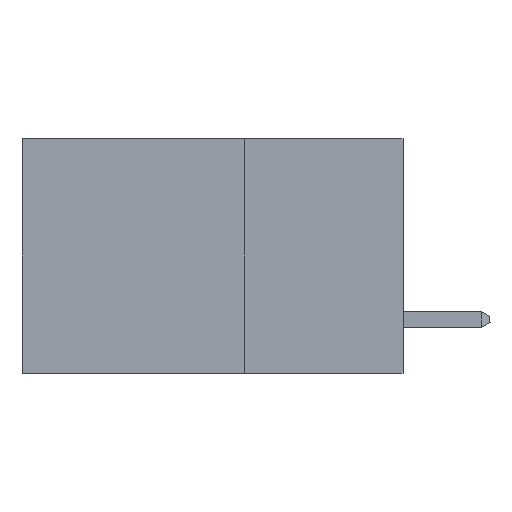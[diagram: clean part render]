
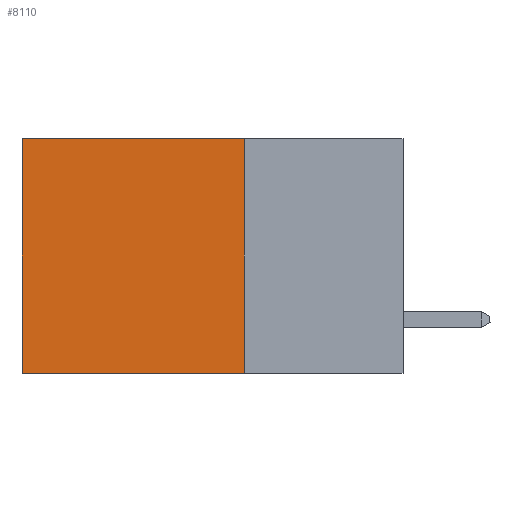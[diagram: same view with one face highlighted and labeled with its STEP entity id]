
A CAD part, left-side view. The second image highlights one B-rep face of the part: STEP entity #8110.
In plain terms, the highlighted planar face has unit normal (-1, 0, 0).
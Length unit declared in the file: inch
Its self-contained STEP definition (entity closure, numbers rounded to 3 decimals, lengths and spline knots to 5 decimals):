
#1140 = EDGE_CURVE ( 'NONE', #17982, #34560, #24422, .T. ) ;
#2813 = CARTESIAN_POINT ( 'NONE',  ( 0.2875, 0.6, -0.37 ) ) ;
#3081 = CARTESIAN_POINT ( 'NONE',  ( 0.2875, 0.25, 0. ) ) ;
#4784 = EDGE_CURVE ( 'NONE', #15243, #38472, #17193, .T. ) ;
#7547 = VECTOR ( 'NONE', #32783, 39.37008 ) ;
#7722 = DIRECTION ( 'NONE',  ( 0., 1., 0. ) ) ;
#8110 = ADVANCED_FACE ( 'NONE', ( #31605 ), #36058, .F. ) ;
#8126 = ORIENTED_EDGE ( 'NONE', *, *, #1140, .T. ) ;
#9093 = ORIENTED_EDGE ( 'NONE', *, *, #23117, .T. ) ;
#9105 = LINE ( 'NONE', #32728, #28887 ) ;
#11068 = CARTESIAN_POINT ( 'NONE',  ( 0.2875, 0.25, 0. ) ) ;
#13843 = CARTESIAN_POINT ( 'NONE',  ( 0.2875, 0.25, 0. ) ) ;
#15006 = CARTESIAN_POINT ( 'NONE',  ( 0.2875, 0.6, 0. ) ) ;
#15243 = VERTEX_POINT ( 'NONE', #29011 ) ;
#17193 = LINE ( 'NONE', #3081, #26628 ) ;
#17982 = VERTEX_POINT ( 'NONE', #27261 ) ;
#18171 = EDGE_LOOP ( 'NONE', ( #8126, #36100, #29002, #9093 ) ) ;
#21955 = EDGE_CURVE ( 'NONE', #38472, #34560, #9105, .T. ) ;
#23117 = EDGE_CURVE ( 'NONE', #15243, #17982, #39137, .T. ) ;
#24422 = LINE ( 'NONE', #15006, #38710 ) ;
#26628 = VECTOR ( 'NONE', #39152, 39.37008 ) ;
#27261 = CARTESIAN_POINT ( 'NONE',  ( 0.2875, 0.6, 0. ) ) ;
#27760 = DIRECTION ( 'NONE',  ( 0., 0., -1. ) ) ;
#28887 = VECTOR ( 'NONE', #7722, 39.37008 ) ;
#29002 = ORIENTED_EDGE ( 'NONE', *, *, #4784, .F. ) ;
#29011 = CARTESIAN_POINT ( 'NONE',  ( 0.2875, 0.25, 0. ) ) ;
#30309 = CARTESIAN_POINT ( 'NONE',  ( 0.2875, 0.25, -0.37 ) ) ;
#31605 = FACE_OUTER_BOUND ( 'NONE', #18171, .T. ) ;
#32728 = CARTESIAN_POINT ( 'NONE',  ( 0.2875, 0.25, -0.37 ) ) ;
#32783 = DIRECTION ( 'NONE',  ( 0., 1., 0. ) ) ;
#34130 = AXIS2_PLACEMENT_3D ( 'NONE', #11068, #36598, #39352 ) ;
#34560 = VERTEX_POINT ( 'NONE', #2813 ) ;
#36058 = PLANE ( 'NONE',  #34130 ) ;
#36100 = ORIENTED_EDGE ( 'NONE', *, *, #21955, .F. ) ;
#36598 = DIRECTION ( 'NONE',  ( 1., 0., 0. ) ) ;
#38472 = VERTEX_POINT ( 'NONE', #30309 ) ;
#38710 = VECTOR ( 'NONE', #27760, 39.37008 ) ;
#39137 = LINE ( 'NONE', #13843, #7547 ) ;
#39152 = DIRECTION ( 'NONE',  ( 0., 0., -1. ) ) ;
#39352 = DIRECTION ( 'NONE',  ( 0., 0., -1. ) ) ;
